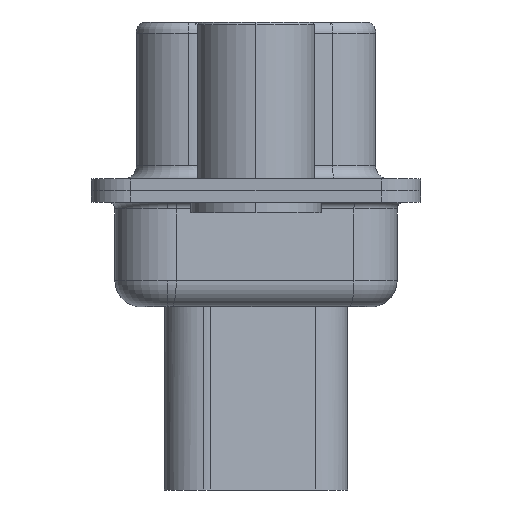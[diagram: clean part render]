
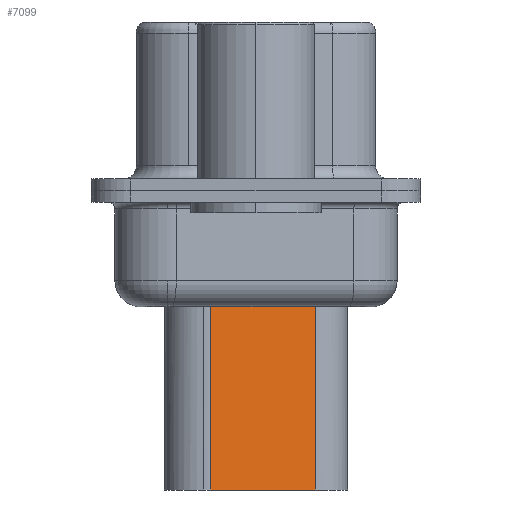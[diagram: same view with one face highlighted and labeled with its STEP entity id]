
A CAD part, left-side view. The second image highlights one B-rep face of the part: STEP entity #7099.
In plain terms, the highlighted planar face has unit normal (-0.985, -0.174, 0).
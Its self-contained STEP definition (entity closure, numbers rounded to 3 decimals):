
#246 = CARTESIAN_POINT ( 'NONE',  ( 4.524, 1.74, -11.45 ) ) ;
#1692 = VERTEX_POINT ( 'NONE', #15596 ) ;
#2320 = ORIENTED_EDGE ( 'NONE', *, *, #5760, .F. ) ;
#2444 = DIRECTION ( 'NONE',  ( 0.174, -0.985, 0. ) ) ;
#3068 = LINE ( 'NONE', #18116, #17194 ) ;
#3806 = VECTOR ( 'NONE', #12291, 1000. ) ;
#3810 = CARTESIAN_POINT ( 'NONE',  ( 5.229, -2.26, -3.1 ) ) ;
#4756 = VERTEX_POINT ( 'NONE', #18460 ) ;
#5760 = EDGE_CURVE ( 'NONE', #1692, #9826, #8343, .T. ) ;
#5767 = EDGE_CURVE ( 'NONE', #1692, #4756, #3068, .T. ) ;
#5973 = CARTESIAN_POINT ( 'NONE',  ( 4.524, 1.74, -3.1 ) ) ;
#6351 = FACE_OUTER_BOUND ( 'NONE', #18782, .T. ) ;
#6872 = LINE ( 'NONE', #22877, #3806 ) ;
#7099 = ADVANCED_FACE ( 'NONE', ( #6351 ), #16561, .T. ) ;
#7535 = DIRECTION ( 'NONE',  ( -0.174, 0.985, 0. ) ) ;
#7949 = EDGE_CURVE ( 'NONE', #4756, #22181, #15469, .T. ) ;
#8343 = LINE ( 'NONE', #3810, #13069 ) ;
#9826 = VERTEX_POINT ( 'NONE', #17137 ) ;
#10956 = DIRECTION ( 'NONE',  ( 0., 0., -1. ) ) ;
#11432 = ORIENTED_EDGE ( 'NONE', *, *, #13482, .F. ) ;
#11803 = CARTESIAN_POINT ( 'NONE',  ( 4.524, 1.74, -3.1 ) ) ;
#12291 = DIRECTION ( 'NONE',  ( -0.174, 0.985, 0. ) ) ;
#13069 = VECTOR ( 'NONE', #10956, 1000. ) ;
#13084 = DIRECTION ( 'NONE',  ( -0.985, -0.174, 0. ) ) ;
#13482 = EDGE_CURVE ( 'NONE', #9826, #22181, #6872, .T. ) ;
#14332 = AXIS2_PLACEMENT_3D ( 'NONE', #5973, #13084, #2444 ) ;
#15469 = LINE ( 'NONE', #11803, #19588 ) ;
#15596 = CARTESIAN_POINT ( 'NONE',  ( 5.229, -2.26, -3.975 ) ) ;
#16561 = PLANE ( 'NONE',  #14332 ) ;
#17137 = CARTESIAN_POINT ( 'NONE',  ( 5.229, -2.26, -11.45 ) ) ;
#17194 = VECTOR ( 'NONE', #7535, 1000. ) ;
#18059 = ORIENTED_EDGE ( 'NONE', *, *, #5767, .T. ) ;
#18116 = CARTESIAN_POINT ( 'NONE',  ( 4.353, 2.709, -3.975 ) ) ;
#18460 = CARTESIAN_POINT ( 'NONE',  ( 4.524, 1.74, -3.975 ) ) ;
#18782 = EDGE_LOOP ( 'NONE', ( #2320, #18059, #21198, #11432 ) ) ;
#19588 = VECTOR ( 'NONE', #22360, 1000. ) ;
#21198 = ORIENTED_EDGE ( 'NONE', *, *, #7949, .T. ) ;
#22181 = VERTEX_POINT ( 'NONE', #246 ) ;
#22360 = DIRECTION ( 'NONE',  ( 0., 0., -1. ) ) ;
#22877 = CARTESIAN_POINT ( 'NONE',  ( 4.524, 1.74, -11.45 ) ) ;
